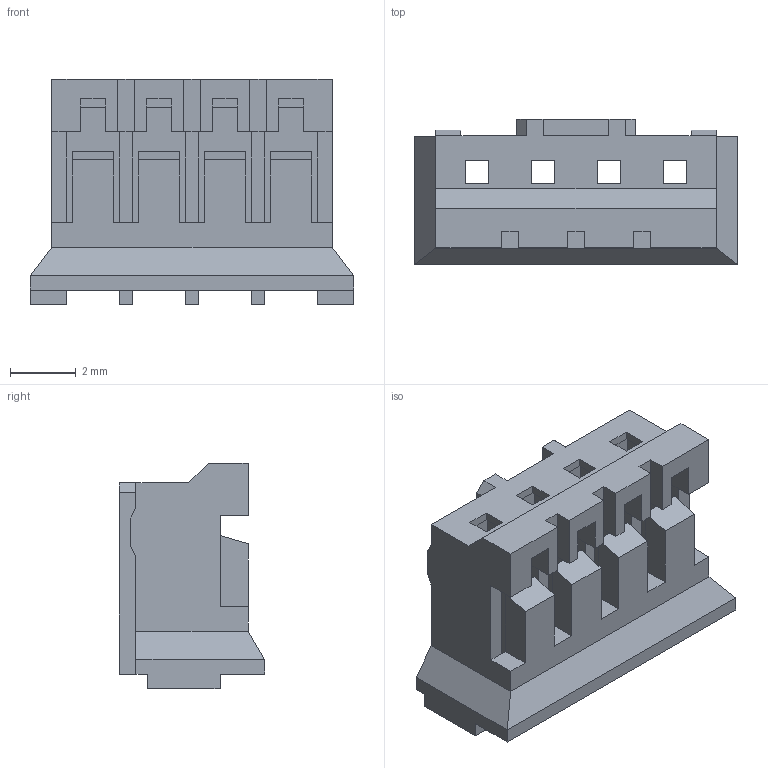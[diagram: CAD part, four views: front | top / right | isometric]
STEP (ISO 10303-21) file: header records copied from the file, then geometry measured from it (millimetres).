
FILE_DESCRIPTION (( 'STEP AP203' ), '1' );
FILE_NAME ('140-504-210-011.STEP', '2020-04-03T13:29:28', ( '' ), ( '' ), 'SwSTEP 2.0', 'SolidWorks 2016', '' );
FILE_SCHEMA (( 'CONFIG_CONTROL_DESIGN' ));
Length unit declared in the file: millimetre
Products named in the file (1): 140-504-210-011
Bounding box: 9.8 x 4.4 x 6.85 mm (x, y, z)
Volume: 98.7 mm3; surface area: 430.3 mm2
Topology: 1 solids, 1 shells, 148 faces, 418 edges, 264 vertices
Faces by surface type: plane 148
Entity records: 4739 total; most frequent: ORIENTED_EDGE 836, CARTESIAN_POINT 831, DIRECTION 716, EDGE_CURVE 418, LINE 418, VECTOR 418, VERTEX_POINT 264, EDGE_LOOP 156
